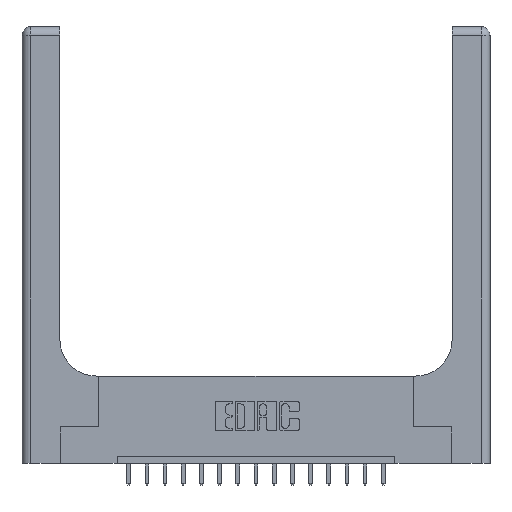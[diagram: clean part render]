
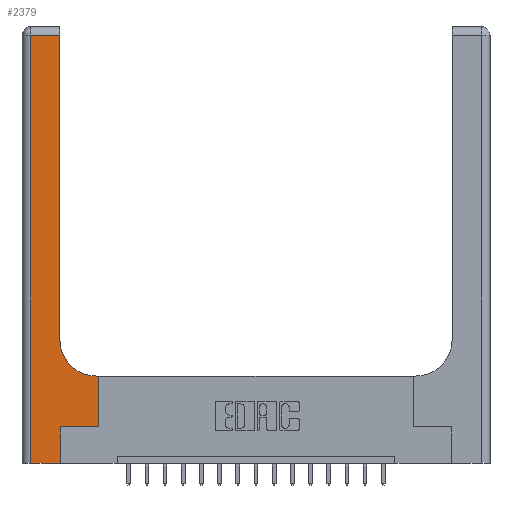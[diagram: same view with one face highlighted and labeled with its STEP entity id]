
A CAD part, top view. The second image highlights one B-rep face of the part: STEP entity #2379.
In plain terms, the highlighted planar face has unit normal (0, 0, 1).
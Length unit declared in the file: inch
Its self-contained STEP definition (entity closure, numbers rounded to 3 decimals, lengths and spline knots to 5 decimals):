
#55 = EDGE_CURVE ( 'NONE', #11926, #6285, #13479, .T. ) ;
#287 = EDGE_CURVE ( 'NONE', #11420, #6101, #1642, .T. ) ;
#384 = VECTOR ( 'NONE', #17174, 39.37008 ) ;
#1020 = DIRECTION ( 'NONE',  ( 1., 0., 0. ) ) ;
#1180 = ORIENTED_EDGE ( 'NONE', *, *, #287, .T. ) ;
#1642 = LINE ( 'NONE', #16097, #4156 ) ;
#1925 = VERTEX_POINT ( 'NONE', #2592 ) ;
#2084 = DIRECTION ( 'NONE',  ( 1., 0., 0. ) ) ;
#2379 = ADVANCED_FACE ( 'NONE', ( #12524 ), #9804, .F. ) ;
#2592 = CARTESIAN_POINT ( 'NONE',  ( 0.26, 0.85, 0.37 ) ) ;
#2782 = CARTESIAN_POINT ( 'NONE',  ( 0.265, 0.25, 0.37 ) ) ;
#3315 = CARTESIAN_POINT ( 'NONE',  ( 0.51, 0.85, 0.37 ) ) ;
#4156 = VECTOR ( 'NONE', #10448, 39.37008 ) ;
#4486 = LINE ( 'NONE', #17185, #9241 ) ;
#4512 = EDGE_CURVE ( 'NONE', #8865, #11926, #7761, .T. ) ;
#4730 = ORIENTED_EDGE ( 'NONE', *, *, #55, .T. ) ;
#4988 = CARTESIAN_POINT ( 'NONE',  ( 0.26, 3., 0.37 ) ) ;
#5177 = DIRECTION ( 'NONE',  ( 0., 1., 0. ) ) ;
#5524 = LINE ( 'NONE', #15385, #9982 ) ;
#5859 = ORIENTED_EDGE ( 'NONE', *, *, #11494, .T. ) ;
#5876 = VERTEX_POINT ( 'NONE', #2782 ) ;
#5891 = CARTESIAN_POINT ( 'NONE',  ( 0., 2.94, 0.37 ) ) ;
#6101 = VERTEX_POINT ( 'NONE', #9805 ) ;
#6285 = VERTEX_POINT ( 'NONE', #8943 ) ;
#6570 = VECTOR ( 'NONE', #6695, 39.37008 ) ;
#6678 = VECTOR ( 'NONE', #11021, 39.37008 ) ;
#6695 = DIRECTION ( 'NONE',  ( 0., -1., 0. ) ) ;
#7490 = DIRECTION ( 'NONE',  ( 0., 1., 0. ) ) ;
#7529 = CARTESIAN_POINT ( 'NONE',  ( 0.528, 0.6, 0.37 ) ) ;
#7565 = EDGE_CURVE ( 'NONE', #1925, #8865, #9226, .T. ) ;
#7761 = LINE ( 'NONE', #5891, #16165 ) ;
#7968 = VERTEX_POINT ( 'NONE', #14622 ) ;
#8028 = AXIS2_PLACEMENT_3D ( 'NONE', #9714, #16951, #12340 ) ;
#8185 = CIRCLE ( 'NONE', #9382, 0.25 ) ;
#8865 = VERTEX_POINT ( 'NONE', #10514 ) ;
#8943 = CARTESIAN_POINT ( 'NONE',  ( 0.06, 0., 0.37 ) ) ;
#9042 = DIRECTION ( 'NONE',  ( 0., 0., -1. ) ) ;
#9122 = EDGE_CURVE ( 'NONE', #6285, #17892, #5524, .T. ) ;
#9217 = EDGE_CURVE ( 'NONE', #5876, #7968, #11464, .T. ) ;
#9226 = LINE ( 'NONE', #4988, #17760 ) ;
#9241 = VECTOR ( 'NONE', #7490, 39.37008 ) ;
#9382 = AXIS2_PLACEMENT_3D ( 'NONE', #3315, #9042, #2084 ) ;
#9510 = LINE ( 'NONE', #16854, #6678 ) ;
#9714 = CARTESIAN_POINT ( 'NONE',  ( 0., 3., 0.37 ) ) ;
#9751 = CARTESIAN_POINT ( 'NONE',  ( 0.265, 0.25, 0.37 ) ) ;
#9804 = PLANE ( 'NONE',  #8028 ) ;
#9805 = CARTESIAN_POINT ( 'NONE',  ( 0.51, 0.6, 0.37 ) ) ;
#9982 = VECTOR ( 'NONE', #1020, 39.37008 ) ;
#10298 = ORIENTED_EDGE ( 'NONE', *, *, #11247, .T. ) ;
#10448 = DIRECTION ( 'NONE',  ( -1., 0., 0. ) ) ;
#10514 = CARTESIAN_POINT ( 'NONE',  ( 0.26, 2.94, 0.37 ) ) ;
#10576 = ORIENTED_EDGE ( 'NONE', *, *, #4512, .T. ) ;
#11021 = DIRECTION ( 'NONE',  ( 0., 1., 0. ) ) ;
#11069 = CARTESIAN_POINT ( 'NONE',  ( 0.06, 2.94, 0.37 ) ) ;
#11247 = EDGE_CURVE ( 'NONE', #17892, #5876, #9510, .T. ) ;
#11420 = VERTEX_POINT ( 'NONE', #7529 ) ;
#11464 = LINE ( 'NONE', #9751, #384 ) ;
#11494 = EDGE_CURVE ( 'NONE', #6101, #1925, #8185, .T. ) ;
#11926 = VERTEX_POINT ( 'NONE', #11069 ) ;
#12340 = DIRECTION ( 'NONE',  ( -1., 0., 0. ) ) ;
#12524 = FACE_OUTER_BOUND ( 'NONE', #16573, .T. ) ;
#13479 = LINE ( 'NONE', #18090, #6570 ) ;
#14423 = ORIENTED_EDGE ( 'NONE', *, *, #16576, .T. ) ;
#14622 = CARTESIAN_POINT ( 'NONE',  ( 0.528, 0.25, 0.37 ) ) ;
#15092 = ORIENTED_EDGE ( 'NONE', *, *, #9217, .T. ) ;
#15302 = ORIENTED_EDGE ( 'NONE', *, *, #7565, .T. ) ;
#15385 = CARTESIAN_POINT ( 'NONE',  ( 0., 0., 0.37 ) ) ;
#16097 = CARTESIAN_POINT ( 'NONE',  ( 0.26, 0.6, 0.37 ) ) ;
#16165 = VECTOR ( 'NONE', #17360, 39.37008 ) ;
#16573 = EDGE_LOOP ( 'NONE', ( #15302, #10576, #4730, #17588, #10298, #15092, #14423, #1180, #5859 ) ) ;
#16576 = EDGE_CURVE ( 'NONE', #7968, #11420, #4486, .T. ) ;
#16854 = CARTESIAN_POINT ( 'NONE',  ( 0.265, 0., 0.37 ) ) ;
#16951 = DIRECTION ( 'NONE',  ( 0., 0., -1. ) ) ;
#16981 = CARTESIAN_POINT ( 'NONE',  ( 0.265, 0., 0.37 ) ) ;
#17174 = DIRECTION ( 'NONE',  ( 1., 0., 0. ) ) ;
#17185 = CARTESIAN_POINT ( 'NONE',  ( 0.528, 0.25, 0.37 ) ) ;
#17360 = DIRECTION ( 'NONE',  ( -1., 0., 0. ) ) ;
#17588 = ORIENTED_EDGE ( 'NONE', *, *, #9122, .T. ) ;
#17760 = VECTOR ( 'NONE', #5177, 39.37008 ) ;
#17892 = VERTEX_POINT ( 'NONE', #16981 ) ;
#18090 = CARTESIAN_POINT ( 'NONE',  ( 0.06, 3., 0.37 ) ) ;
